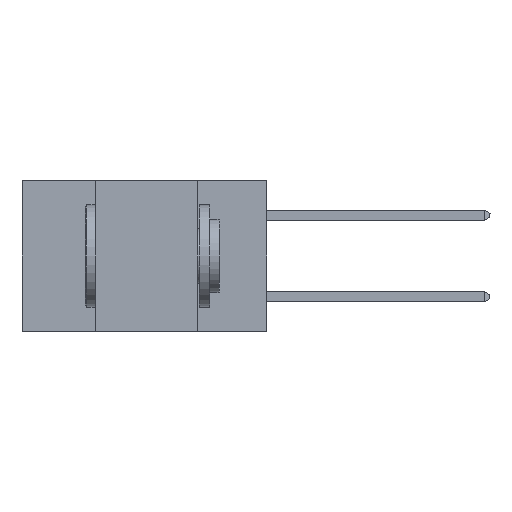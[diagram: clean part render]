
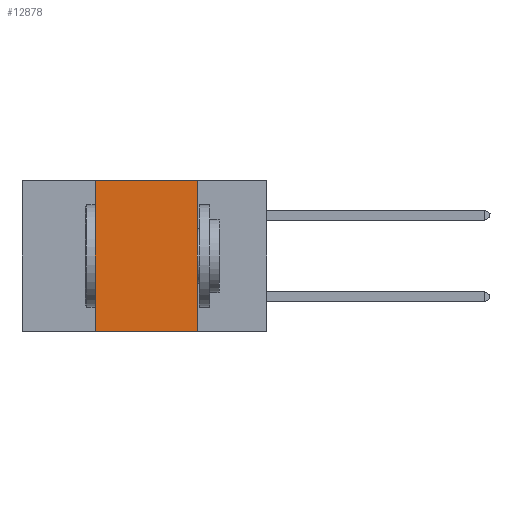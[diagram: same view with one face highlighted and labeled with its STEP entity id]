
A CAD part, left-side view. The second image highlights one B-rep face of the part: STEP entity #12878.
In plain terms, the highlighted planar face has unit normal (-1, 0, 0).
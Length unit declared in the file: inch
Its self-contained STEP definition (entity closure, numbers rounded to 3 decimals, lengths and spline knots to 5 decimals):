
#465 = CARTESIAN_POINT ( 'NONE',  ( 0., 0.17, 0. ) ) ;
#474 = DIRECTION ( 'NONE',  ( 0., 0., 1. ) ) ;
#530 = CARTESIAN_POINT ( 'NONE',  ( 0., 0.42, 0. ) ) ;
#640 = EDGE_CURVE ( 'NONE', #9310, #9303, #16041, .T. ) ;
#708 = CARTESIAN_POINT ( 'NONE',  ( 0., 0.42, -0.37 ) ) ;
#756 = ORIENTED_EDGE ( 'NONE', *, *, #640, .T. ) ;
#1716 = LINE ( 'NONE', #465, #3643 ) ;
#2397 = LINE ( 'NONE', #8761, #10635 ) ;
#3250 = DIRECTION ( 'NONE',  ( 0., 0., -1. ) ) ;
#3643 = VECTOR ( 'NONE', #5147, 39.37008 ) ;
#3994 = AXIS2_PLACEMENT_3D ( 'NONE', #12428, #12549, #3250 ) ;
#5147 = DIRECTION ( 'NONE',  ( 0., 0., -1. ) ) ;
#5154 = CARTESIAN_POINT ( 'NONE',  ( 0., 0.42, 0. ) ) ;
#5381 = EDGE_LOOP ( 'NONE', ( #12824, #9356, #5437, #756 ) ) ;
#5437 = ORIENTED_EDGE ( 'NONE', *, *, #9885, .F. ) ;
#7504 = EDGE_CURVE ( 'NONE', #9511, #9303, #1716, .T. ) ;
#7853 = PLANE ( 'NONE',  #3994 ) ;
#8761 = CARTESIAN_POINT ( 'NONE',  ( 0., 0.6, 0. ) ) ;
#9303 = VERTEX_POINT ( 'NONE', #10704 ) ;
#9310 = VERTEX_POINT ( 'NONE', #708 ) ;
#9356 = ORIENTED_EDGE ( 'NONE', *, *, #13923, .F. ) ;
#9511 = VERTEX_POINT ( 'NONE', #9751 ) ;
#9751 = CARTESIAN_POINT ( 'NONE',  ( 0., 0.17, 0. ) ) ;
#9885 = EDGE_CURVE ( 'NONE', #9310, #15001, #15729, .T. ) ;
#10635 = VECTOR ( 'NONE', #19435, 39.37008 ) ;
#10704 = CARTESIAN_POINT ( 'NONE',  ( 0., 0.17, -0.37 ) ) ;
#11591 = VECTOR ( 'NONE', #474, 39.37008 ) ;
#12428 = CARTESIAN_POINT ( 'NONE',  ( 0., 0.6, 0. ) ) ;
#12549 = DIRECTION ( 'NONE',  ( 1., 0., 0. ) ) ;
#12824 = ORIENTED_EDGE ( 'NONE', *, *, #7504, .F. ) ;
#12878 = ADVANCED_FACE ( 'NONE', ( #17221 ), #7853, .F. ) ;
#13923 = EDGE_CURVE ( 'NONE', #15001, #9511, #2397, .T. ) ;
#15001 = VERTEX_POINT ( 'NONE', #530 ) ;
#15729 = LINE ( 'NONE', #5154, #11591 ) ;
#16041 = LINE ( 'NONE', #19989, #18251 ) ;
#16937 = DIRECTION ( 'NONE',  ( 0., -1., 0. ) ) ;
#17221 = FACE_OUTER_BOUND ( 'NONE', #5381, .T. ) ;
#18251 = VECTOR ( 'NONE', #16937, 39.37008 ) ;
#19435 = DIRECTION ( 'NONE',  ( 0., -1., 0. ) ) ;
#19989 = CARTESIAN_POINT ( 'NONE',  ( 0., 0.6, -0.37 ) ) ;
